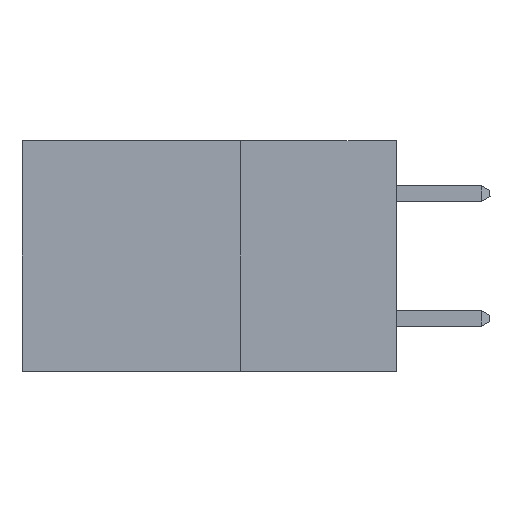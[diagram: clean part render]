
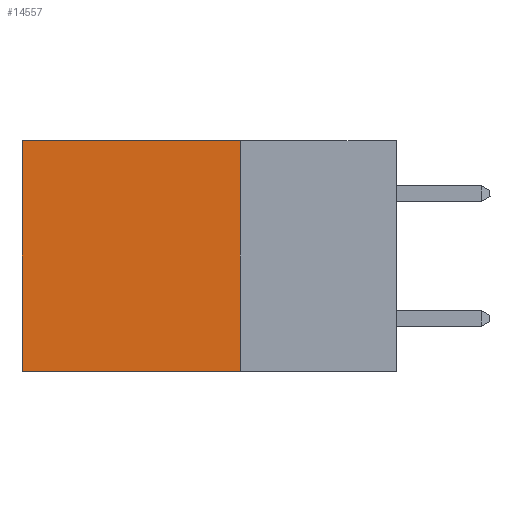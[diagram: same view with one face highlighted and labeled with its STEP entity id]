
A CAD part, left-side view. The second image highlights one B-rep face of the part: STEP entity #14557.
In plain terms, the highlighted planar face has unit normal (-1, 0, 0).
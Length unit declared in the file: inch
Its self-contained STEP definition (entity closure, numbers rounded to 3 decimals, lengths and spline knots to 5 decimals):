
#1692 = CARTESIAN_POINT ( 'NONE',  ( 0.298, 0.25, 0. ) ) ;
#2024 = ORIENTED_EDGE ( 'NONE', *, *, #8111, .F. ) ;
#2597 = PLANE ( 'NONE',  #25926 ) ;
#4558 = EDGE_CURVE ( 'NONE', #9044, #22100, #9326, .T. ) ;
#5366 = CARTESIAN_POINT ( 'NONE',  ( 0.298, 0.25, -0.37 ) ) ;
#5705 = CARTESIAN_POINT ( 'NONE',  ( 0.298, 0.25, 0. ) ) ;
#5804 = VECTOR ( 'NONE', #18581, 39.37008 ) ;
#6816 = CARTESIAN_POINT ( 'NONE',  ( 0.298, 0.25, 0. ) ) ;
#7864 = DIRECTION ( 'NONE',  ( 0., 0., -1. ) ) ;
#8111 = EDGE_CURVE ( 'NONE', #22100, #24951, #12929, .T. ) ;
#8485 = ORIENTED_EDGE ( 'NONE', *, *, #4558, .F. ) ;
#9009 = VECTOR ( 'NONE', #7864, 39.37008 ) ;
#9044 = VERTEX_POINT ( 'NONE', #6816 ) ;
#9326 = LINE ( 'NONE', #5705, #9009 ) ;
#10332 = FACE_OUTER_BOUND ( 'NONE', #16354, .T. ) ;
#11055 = VECTOR ( 'NONE', #27238, 39.37008 ) ;
#12007 = EDGE_CURVE ( 'NONE', #23285, #24951, #16143, .T. ) ;
#12228 = ORIENTED_EDGE ( 'NONE', *, *, #12007, .T. ) ;
#12289 = CARTESIAN_POINT ( 'NONE',  ( 0.298, 0.6, 0. ) ) ;
#12929 = LINE ( 'NONE', #27357, #5804 ) ;
#13121 = CARTESIAN_POINT ( 'NONE',  ( 0.298, 0.25, 0. ) ) ;
#13305 = LINE ( 'NONE', #1692, #18768 ) ;
#13414 = DIRECTION ( 'NONE',  ( 1., 0., 0. ) ) ;
#14557 = ADVANCED_FACE ( 'NONE', ( #10332 ), #2597, .F. ) ;
#15067 = EDGE_CURVE ( 'NONE', #9044, #23285, #13305, .T. ) ;
#16143 = LINE ( 'NONE', #12289, #11055 ) ;
#16354 = EDGE_LOOP ( 'NONE', ( #12228, #2024, #8485, #24956 ) ) ;
#18581 = DIRECTION ( 'NONE',  ( 0., 1., 0. ) ) ;
#18768 = VECTOR ( 'NONE', #23036, 39.37008 ) ;
#22100 = VERTEX_POINT ( 'NONE', #5366 ) ;
#23036 = DIRECTION ( 'NONE',  ( 0., 1., 0. ) ) ;
#23285 = VERTEX_POINT ( 'NONE', #23704 ) ;
#23704 = CARTESIAN_POINT ( 'NONE',  ( 0.298, 0.6, 0. ) ) ;
#24328 = CARTESIAN_POINT ( 'NONE',  ( 0.298, 0.6, -0.37 ) ) ;
#24951 = VERTEX_POINT ( 'NONE', #24328 ) ;
#24956 = ORIENTED_EDGE ( 'NONE', *, *, #15067, .T. ) ;
#25926 = AXIS2_PLACEMENT_3D ( 'NONE', #13121, #13414, #26183 ) ;
#26183 = DIRECTION ( 'NONE',  ( 0., 0., -1. ) ) ;
#27238 = DIRECTION ( 'NONE',  ( 0., 0., -1. ) ) ;
#27357 = CARTESIAN_POINT ( 'NONE',  ( 0.298, 0.25, -0.37 ) ) ;
